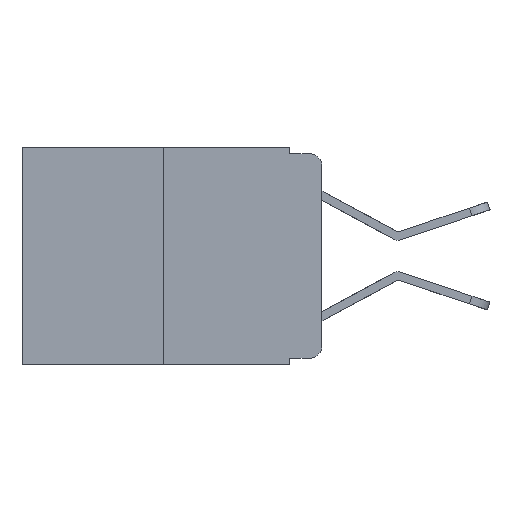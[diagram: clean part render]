
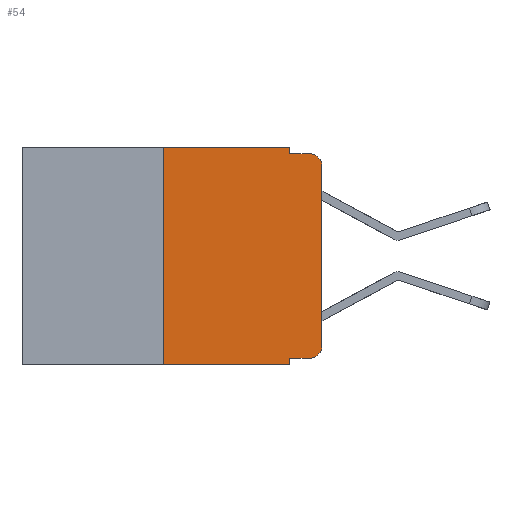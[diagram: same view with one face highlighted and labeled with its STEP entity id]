
A CAD part, left-side view. The second image highlights one B-rep face of the part: STEP entity #54.
In plain terms, the highlighted planar face has unit normal (-1, 0, 0).
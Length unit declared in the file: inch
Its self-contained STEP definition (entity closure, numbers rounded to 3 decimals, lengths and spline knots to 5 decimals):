
#54 = ADVANCED_FACE ( 'NONE', ( #5878 ), #17605, .F. ) ;
#650 = CARTESIAN_POINT ( 'NONE',  ( 0., 0., -0.313 ) ) ;
#1022 = EDGE_CURVE ( 'NONE', #10283, #7625, #3285, .T. ) ;
#1260 = LINE ( 'NONE', #16362, #19176 ) ;
#1597 = VERTEX_POINT ( 'NONE', #2001 ) ;
#2001 = CARTESIAN_POINT ( 'NONE',  ( 0., 0.051, -0.01 ) ) ;
#2117 = VECTOR ( 'NONE', #6281, 39.37008 ) ;
#2586 = VERTEX_POINT ( 'NONE', #20864 ) ;
#2680 = LINE ( 'NONE', #17645, #17940 ) ;
#3140 = LINE ( 'NONE', #8012, #16337 ) ;
#3285 = LINE ( 'NONE', #6205, #2117 ) ;
#3570 = EDGE_CURVE ( 'NONE', #7625, #18978, #8722, .T. ) ;
#3687 = DIRECTION ( 'NONE',  ( -1., 0., 0. ) ) ;
#4258 = CARTESIAN_POINT ( 'NONE',  ( 0., 0.25, -0.343 ) ) ;
#4408 = ORIENTED_EDGE ( 'NONE', *, *, #20795, .F. ) ;
#4650 = VERTEX_POINT ( 'NONE', #4258 ) ;
#4765 = EDGE_CURVE ( 'NONE', #1597, #18978, #3140, .T. ) ;
#4960 = ORIENTED_EDGE ( 'NONE', *, *, #21779, .T. ) ;
#5079 = EDGE_CURVE ( 'NONE', #13671, #10283, #15534, .T. ) ;
#5587 = CARTESIAN_POINT ( 'NONE',  ( 0., 0.051, 0. ) ) ;
#5745 = DIRECTION ( 'NONE',  ( 0., 0., 1. ) ) ;
#5878 = FACE_OUTER_BOUND ( 'NONE', #15761, .T. ) ;
#6104 = LINE ( 'NONE', #5587, #19141 ) ;
#6205 = CARTESIAN_POINT ( 'NONE',  ( 0., 0., 0. ) ) ;
#6281 = DIRECTION ( 'NONE',  ( 0., 0., 1. ) ) ;
#6699 = EDGE_CURVE ( 'NONE', #10625, #13671, #1260, .T. ) ;
#6711 = VERTEX_POINT ( 'NONE', #7999 ) ;
#6832 = VECTOR ( 'NONE', #8879, 39.37008 ) ;
#7166 = CARTESIAN_POINT ( 'NONE',  ( 0., 0.473, 0. ) ) ;
#7625 = VERTEX_POINT ( 'NONE', #17596 ) ;
#7828 = VECTOR ( 'NONE', #15134, 39.37008 ) ;
#7999 = CARTESIAN_POINT ( 'NONE',  ( 0., 0.25, 0. ) ) ;
#8012 = CARTESIAN_POINT ( 'NONE',  ( 0., 0.051, -0.01 ) ) ;
#8051 = CARTESIAN_POINT ( 'NONE',  ( 0., 0.02, -0.03 ) ) ;
#8087 = VECTOR ( 'NONE', #12235, 39.37008 ) ;
#8274 = EDGE_CURVE ( 'NONE', #2586, #1597, #6104, .T. ) ;
#8492 = CARTESIAN_POINT ( 'NONE',  ( 0., 0.473, -0.343 ) ) ;
#8722 = CIRCLE ( 'NONE', #19161, 0.02 ) ;
#8794 = CARTESIAN_POINT ( 'NONE',  ( 0., 0.051, 0. ) ) ;
#8879 = DIRECTION ( 'NONE',  ( 0., -1., 0. ) ) ;
#9792 = DIRECTION ( 'NONE',  ( 0., 0., -1. ) ) ;
#10283 = VERTEX_POINT ( 'NONE', #650 ) ;
#10625 = VERTEX_POINT ( 'NONE', #18905 ) ;
#10820 = DIRECTION ( 'NONE',  ( 0., 0., -1. ) ) ;
#11334 = LINE ( 'NONE', #8492, #7828 ) ;
#12056 = AXIS2_PLACEMENT_3D ( 'NONE', #15118, #18182, #17826 ) ;
#12235 = DIRECTION ( 'NONE',  ( 0., 0., -1. ) ) ;
#12409 = CARTESIAN_POINT ( 'NONE',  ( 0., 0.02, -0.01 ) ) ;
#12523 = AXIS2_PLACEMENT_3D ( 'NONE', #13993, #3687, #15694 ) ;
#13035 = ORIENTED_EDGE ( 'NONE', *, *, #5079, .T. ) ;
#13492 = ORIENTED_EDGE ( 'NONE', *, *, #1022, .T. ) ;
#13671 = VERTEX_POINT ( 'NONE', #19437 ) ;
#13993 = CARTESIAN_POINT ( 'NONE',  ( 0., 0.02, -0.313 ) ) ;
#14177 = CARTESIAN_POINT ( 'NONE',  ( 0., 0.051, -0.343 ) ) ;
#14649 = DIRECTION ( 'NONE',  ( 0., -1., 0. ) ) ;
#14814 = ORIENTED_EDGE ( 'NONE', *, *, #8274, .F. ) ;
#15118 = CARTESIAN_POINT ( 'NONE',  ( 0., 0.473, 0. ) ) ;
#15134 = DIRECTION ( 'NONE',  ( 0., -1., 0. ) ) ;
#15534 = CIRCLE ( 'NONE', #12523, 0.02 ) ;
#15694 = DIRECTION ( 'NONE',  ( 0., 0., -1. ) ) ;
#15761 = EDGE_LOOP ( 'NONE', ( #13492, #16139, #16652, #14814, #18276, #4408, #4960, #22312, #15936, #13035 ) ) ;
#15936 = ORIENTED_EDGE ( 'NONE', *, *, #6699, .T. ) ;
#16139 = ORIENTED_EDGE ( 'NONE', *, *, #3570, .T. ) ;
#16337 = VECTOR ( 'NONE', #21572, 39.37008 ) ;
#16362 = CARTESIAN_POINT ( 'NONE',  ( 0., 0.051, -0.333 ) ) ;
#16652 = ORIENTED_EDGE ( 'NONE', *, *, #4765, .F. ) ;
#16978 = EDGE_CURVE ( 'NONE', #6711, #2586, #20391, .T. ) ;
#17596 = CARTESIAN_POINT ( 'NONE',  ( 0., 0., -0.03 ) ) ;
#17605 = PLANE ( 'NONE',  #12056 ) ;
#17645 = CARTESIAN_POINT ( 'NONE',  ( 0., 0.25, 0. ) ) ;
#17826 = DIRECTION ( 'NONE',  ( 0., 0., -1. ) ) ;
#17940 = VECTOR ( 'NONE', #5745, 39.37008 ) ;
#18182 = DIRECTION ( 'NONE',  ( 1., 0., 0. ) ) ;
#18276 = ORIENTED_EDGE ( 'NONE', *, *, #16978, .F. ) ;
#18905 = CARTESIAN_POINT ( 'NONE',  ( 0., 0.051, -0.333 ) ) ;
#18978 = VERTEX_POINT ( 'NONE', #12409 ) ;
#19141 = VECTOR ( 'NONE', #10820, 39.37008 ) ;
#19161 = AXIS2_PLACEMENT_3D ( 'NONE', #8051, #19924, #9792 ) ;
#19176 = VECTOR ( 'NONE', #14649, 39.37008 ) ;
#19437 = CARTESIAN_POINT ( 'NONE',  ( 0., 0.02, -0.333 ) ) ;
#19924 = DIRECTION ( 'NONE',  ( -1., 0., 0. ) ) ;
#20302 = VERTEX_POINT ( 'NONE', #14177 ) ;
#20391 = LINE ( 'NONE', #7166, #6832 ) ;
#20795 = EDGE_CURVE ( 'NONE', #4650, #6711, #2680, .T. ) ;
#20864 = CARTESIAN_POINT ( 'NONE',  ( 0., 0.051, 0. ) ) ;
#21572 = DIRECTION ( 'NONE',  ( 0., -1., 0. ) ) ;
#21610 = LINE ( 'NONE', #8794, #8087 ) ;
#21779 = EDGE_CURVE ( 'NONE', #4650, #20302, #11334, .T. ) ;
#21922 = EDGE_CURVE ( 'NONE', #10625, #20302, #21610, .T. ) ;
#22312 = ORIENTED_EDGE ( 'NONE', *, *, #21922, .F. ) ;
